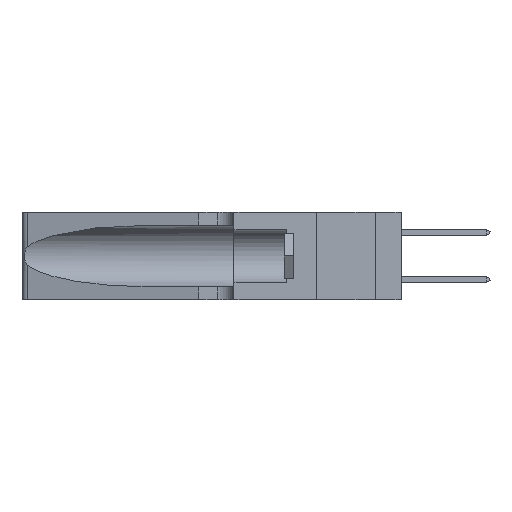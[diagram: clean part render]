
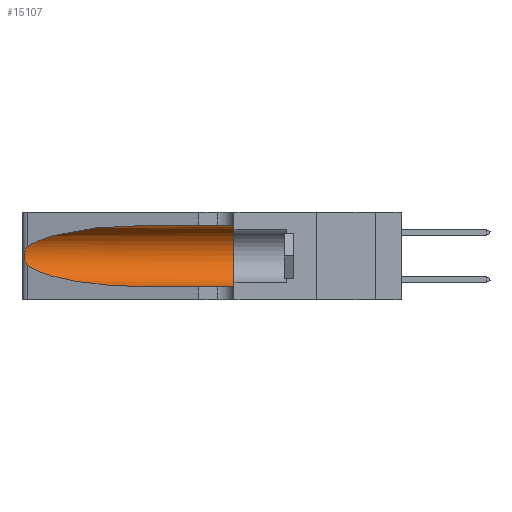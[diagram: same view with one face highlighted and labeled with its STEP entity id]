
A CAD part, left-side view. The second image highlights one B-rep face of the part: STEP entity #15107.
In plain terms, the highlighted cylindrical face has radius 3.308 mm (diameter 6.617 mm), a partial arc.
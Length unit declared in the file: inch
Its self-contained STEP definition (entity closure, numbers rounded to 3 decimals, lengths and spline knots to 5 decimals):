
#1643 = VERTEX_POINT ( 'NONE', #19548 ) ;
#3028 = CARTESIAN_POINT ( 'NONE',  ( 0.1305, 1.61858, 0.31525 ) ) ;
#3051 = EDGE_CURVE ( 'NONE', #1643, #15328, #21572, .T. ) ;
#3410 = CARTESIAN_POINT ( 'NONE',  ( 0.26075, 1.23896, 0.19203 ) ) ;
#4394 = VERTEX_POINT ( 'NONE', #34396 ) ;
#6570 = VECTOR ( 'NONE', #42105, 39.37008 ) ;
#7171 = CARTESIAN_POINT ( 'NONE',  ( 0.25789, 1.23486, 0.15765 ) ) ;
#7522 = EDGE_CURVE ( 'NONE', #1643, #11447, #23078, .T. ) ;
#7804 = CARTESIAN_POINT ( 'NONE',  ( 0.25639, 1.23184, 0.21858 ) ) ;
#7832 = EDGE_CURVE ( 'NONE', #21497, #23042, #25176, .T. ) ;
#8377 = CARTESIAN_POINT ( 'NONE',  ( 0.1305, 0.72297, 0.05475 ) ) ;
#8931 = CARTESIAN_POINT ( 'NONE',  ( 0.1305, 0.72297, 0.31525 ) ) ;
#9689 = EDGE_CURVE ( 'NONE', #23042, #4394, #14064, .T. ) ;
#11447 = VERTEX_POINT ( 'NONE', #15549 ) ;
#11503 = CARTESIAN_POINT ( 'NONE',  ( 0.25639, 1.23186, 0.15144 ) ) ;
#13160 = VECTOR ( 'NONE', #14828, 39.37008 ) ;
#14064 = LINE ( 'NONE', #42255, #6570 ) ;
#14828 = DIRECTION ( 'NONE',  ( 0., -1., 0. ) ) ;
#14895 = CARTESIAN_POINT ( 'NONE',  ( 0.25555, 1.22993, 0.14849 ) ) ;
#15107 = ADVANCED_FACE ( 'NONE', ( #17254 ), #35977, .F. ) ;
#15328 = VERTEX_POINT ( 'NONE', #43165 ) ;
#15549 = CARTESIAN_POINT ( 'NONE',  ( 0.1305, 0.35, 0.31525 ) ) ;
#15708 = CARTESIAN_POINT ( 'NONE',  ( 0.2373, 1.15595, 0.28018 ) ) ;
#16839 = CARTESIAN_POINT ( 'NONE',  ( 0.25487, 1.22718, 0.22369 ) ) ;
#17254 = FACE_OUTER_BOUND ( 'NONE', #30838, .T. ) ;
#17962 = B_SPLINE_CURVE_WITH_KNOTS ( 'NONE', 3,
 ( #18644, #26347, #7804, #37425, #33856, #36951, #3410, #29473, #44954, #22574, #7171, #11503, #14895, #22398 ),
 .UNSPECIFIED., .F., .F.,
 ( 4, 2, 2, 2, 2, 2, 4 ),
 ( 0., 0.00027, 0.00053, 0.00107, 0.0016, 0.00187, 0.00214 ),
 .UNSPECIFIED. ) ;
#18644 = CARTESIAN_POINT ( 'NONE',  ( 0.25487, 1.22718, 0.22369 ) ) ;
#19386 = CARTESIAN_POINT ( 'NONE',  ( 0.25487, 1.22718, 0.14631 ) ) ;
#19548 = CARTESIAN_POINT ( 'NONE',  ( 0.1305, 0.72297, 0.31525 ) ) ;
#20372 = AXIS2_PLACEMENT_3D ( 'NONE', #41702, #30634, #23257 ) ;
#20672 = AXIS2_PLACEMENT_3D ( 'NONE', #33101, #26868, #34545 ) ;
#21497 = VERTEX_POINT ( 'NONE', #30768 ) ;
#21572 =( BOUNDED_CURVE ( )  B_SPLINE_CURVE ( 3, ( #8931, #38113, #15708, #16839 ),
 .UNSPECIFIED., .F., .T. ) 
 B_SPLINE_CURVE_WITH_KNOTS ( ( 4, 4 ),
 ( 1.5708, 2.84003 ),
 .UNSPECIFIED. ) 
 CURVE ( )  GEOMETRIC_REPRESENTATION_ITEM ( )  RATIONAL_B_SPLINE_CURVE ( ( 1., 0.87, 0.87, 1. ) ) 
 REPRESENTATION_ITEM ( '' )  );
#22398 = CARTESIAN_POINT ( 'NONE',  ( 0.25487, 1.22718, 0.14631 ) ) ;
#22574 = CARTESIAN_POINT ( 'NONE',  ( 0.25856, 1.23593, 0.16098 ) ) ;
#23042 = VERTEX_POINT ( 'NONE', #23474 ) ;
#23078 = LINE ( 'NONE', #3028, #13160 ) ;
#23257 = DIRECTION ( 'NONE',  ( 0., 0., -1. ) ) ;
#23281 = ORIENTED_EDGE ( 'NONE', *, *, #7522, .F. ) ;
#23474 = CARTESIAN_POINT ( 'NONE',  ( 0.1305, 0.72297, 0.05475 ) ) ;
#25176 =( BOUNDED_CURVE ( )  B_SPLINE_CURVE ( 3, ( #19386, #45852, #34777, #8377 ),
 .UNSPECIFIED., .F., .T. ) 
 B_SPLINE_CURVE_WITH_KNOTS ( ( 4, 4 ),
 ( 3.44316, 4.71239 ),
 .UNSPECIFIED. ) 
 CURVE ( )  GEOMETRIC_REPRESENTATION_ITEM ( )  RATIONAL_B_SPLINE_CURVE ( ( 1., 0.87, 0.87, 1. ) ) 
 REPRESENTATION_ITEM ( '' )  );
#26347 = CARTESIAN_POINT ( 'NONE',  ( 0.25555, 1.22994, 0.2215 ) ) ;
#26868 = DIRECTION ( 'NONE',  ( 0., 1., 0. ) ) ;
#28520 = EDGE_CURVE ( 'NONE', #15328, #21497, #17962, .T. ) ;
#29473 = CARTESIAN_POINT ( 'NONE',  ( 0.26075, 1.23896, 0.178 ) ) ;
#30634 = DIRECTION ( 'NONE',  ( 0., -1., 0. ) ) ;
#30768 = CARTESIAN_POINT ( 'NONE',  ( 0.25487, 1.22718, 0.14631 ) ) ;
#30838 = EDGE_LOOP ( 'NONE', ( #47584, #42488, #44028, #37963, #33880, #23281 ) ) ;
#33101 = CARTESIAN_POINT ( 'NONE',  ( 0.1305, 0.35, 0.185 ) ) ;
#33856 = CARTESIAN_POINT ( 'NONE',  ( 0.25854, 1.2359, 0.20912 ) ) ;
#33880 = ORIENTED_EDGE ( 'NONE', *, *, #35932, .F. ) ;
#34396 = CARTESIAN_POINT ( 'NONE',  ( 0.1305, 0.35, 0.05475 ) ) ;
#34545 = DIRECTION ( 'NONE',  ( 0., 0., 1. ) ) ;
#34777 = CARTESIAN_POINT ( 'NONE',  ( 0.18966, 0.96281, 0.05475 ) ) ;
#35932 = EDGE_CURVE ( 'NONE', #11447, #4394, #47226, .T. ) ;
#35977 = CYLINDRICAL_SURFACE ( 'NONE', #20372, 0.13025 ) ;
#36951 = CARTESIAN_POINT ( 'NONE',  ( 0.26018, 1.23835, 0.19895 ) ) ;
#37425 = CARTESIAN_POINT ( 'NONE',  ( 0.25787, 1.23484, 0.2124 ) ) ;
#37963 = ORIENTED_EDGE ( 'NONE', *, *, #9689, .T. ) ;
#38113 = CARTESIAN_POINT ( 'NONE',  ( 0.18966, 0.96281, 0.31525 ) ) ;
#41702 = CARTESIAN_POINT ( 'NONE',  ( 0.1305, 1.61858, 0.185 ) ) ;
#42105 = DIRECTION ( 'NONE',  ( 0., -1., 0. ) ) ;
#42255 = CARTESIAN_POINT ( 'NONE',  ( 0.1305, 1.61858, 0.05475 ) ) ;
#42488 = ORIENTED_EDGE ( 'NONE', *, *, #28520, .T. ) ;
#43165 = CARTESIAN_POINT ( 'NONE',  ( 0.25487, 1.22718, 0.22369 ) ) ;
#44028 = ORIENTED_EDGE ( 'NONE', *, *, #7832, .T. ) ;
#44954 = CARTESIAN_POINT ( 'NONE',  ( 0.26017, 1.23833, 0.17102 ) ) ;
#45852 = CARTESIAN_POINT ( 'NONE',  ( 0.2373, 1.15595, 0.08982 ) ) ;
#47226 = CIRCLE ( 'NONE', #20672, 0.13025 ) ;
#47584 = ORIENTED_EDGE ( 'NONE', *, *, #3051, .T. ) ;
